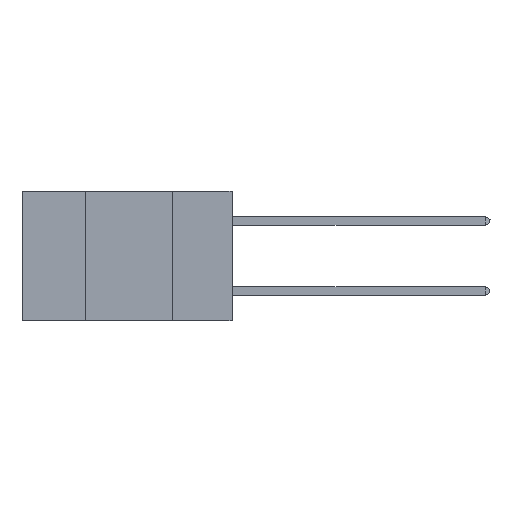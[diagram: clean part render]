
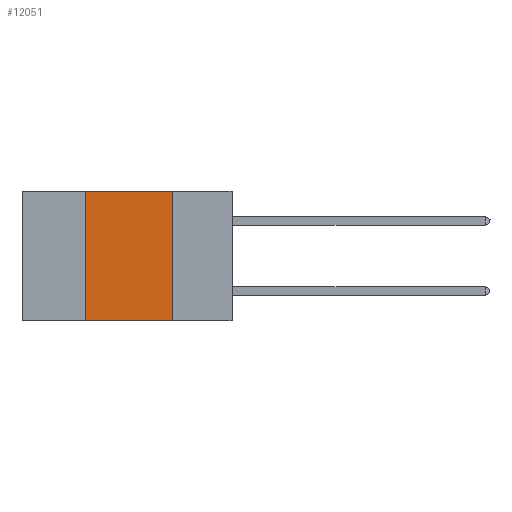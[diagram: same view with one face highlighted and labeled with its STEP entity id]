
A CAD part, left-side view. The second image highlights one B-rep face of the part: STEP entity #12051.
In plain terms, the highlighted planar face has unit normal (-1, 0, 0).
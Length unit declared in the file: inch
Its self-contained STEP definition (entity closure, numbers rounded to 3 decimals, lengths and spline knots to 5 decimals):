
#187 = ORIENTED_EDGE ( 'NONE', *, *, #6184, .F. ) ;
#959 = VERTEX_POINT ( 'NONE', #13045 ) ;
#1381 = DIRECTION ( 'NONE',  ( 1., 0., 0. ) ) ;
#6157 = LINE ( 'NONE', #16848, #11087 ) ;
#6184 = EDGE_CURVE ( 'NONE', #10202, #10381, #16289, .T. ) ;
#6401 = LINE ( 'NONE', #16070, #16402 ) ;
#6920 = DIRECTION ( 'NONE',  ( 0., 0., 1. ) ) ;
#7914 = EDGE_CURVE ( 'NONE', #10202, #959, #6401, .T. ) ;
#7985 = DIRECTION ( 'NONE',  ( 0., 0., -1. ) ) ;
#8588 = LINE ( 'NONE', #16105, #8803 ) ;
#8803 = VECTOR ( 'NONE', #13298, 39.37008 ) ;
#9002 = AXIS2_PLACEMENT_3D ( 'NONE', #14045, #1381, #7985 ) ;
#9025 = DIRECTION ( 'NONE',  ( 0., -1., 0. ) ) ;
#9211 = FACE_OUTER_BOUND ( 'NONE', #19180, .T. ) ;
#9311 = PLANE ( 'NONE',  #9002 ) ;
#10099 = CARTESIAN_POINT ( 'NONE',  ( 0., 0.42, 0. ) ) ;
#10202 = VERTEX_POINT ( 'NONE', #14899 ) ;
#10381 = VERTEX_POINT ( 'NONE', #10099 ) ;
#11087 = VECTOR ( 'NONE', #9025, 39.37008 ) ;
#12051 = ADVANCED_FACE ( 'NONE', ( #9211 ), #9311, .F. ) ;
#12653 = DIRECTION ( 'NONE',  ( 0., -1., 0. ) ) ;
#12728 = ORIENTED_EDGE ( 'NONE', *, *, #19046, .F. ) ;
#13045 = CARTESIAN_POINT ( 'NONE',  ( 0., 0.17, -0.37 ) ) ;
#13298 = DIRECTION ( 'NONE',  ( 0., 0., -1. ) ) ;
#13891 = VECTOR ( 'NONE', #6920, 39.37008 ) ;
#13928 = ORIENTED_EDGE ( 'NONE', *, *, #19760, .F. ) ;
#14045 = CARTESIAN_POINT ( 'NONE',  ( 0., 0.6, 0. ) ) ;
#14847 = CARTESIAN_POINT ( 'NONE',  ( 0., 0.42, 0. ) ) ;
#14899 = CARTESIAN_POINT ( 'NONE',  ( 0., 0.42, -0.37 ) ) ;
#14913 = VERTEX_POINT ( 'NONE', #18396 ) ;
#16070 = CARTESIAN_POINT ( 'NONE',  ( 0., 0.6, -0.37 ) ) ;
#16105 = CARTESIAN_POINT ( 'NONE',  ( 0., 0.17, 0. ) ) ;
#16289 = LINE ( 'NONE', #14847, #13891 ) ;
#16402 = VECTOR ( 'NONE', #12653, 39.37008 ) ;
#16848 = CARTESIAN_POINT ( 'NONE',  ( 0., 0.6, 0. ) ) ;
#17074 = ORIENTED_EDGE ( 'NONE', *, *, #7914, .T. ) ;
#18396 = CARTESIAN_POINT ( 'NONE',  ( 0., 0.17, 0. ) ) ;
#19046 = EDGE_CURVE ( 'NONE', #10381, #14913, #6157, .T. ) ;
#19180 = EDGE_LOOP ( 'NONE', ( #13928, #12728, #187, #17074 ) ) ;
#19760 = EDGE_CURVE ( 'NONE', #14913, #959, #8588, .T. ) ;
